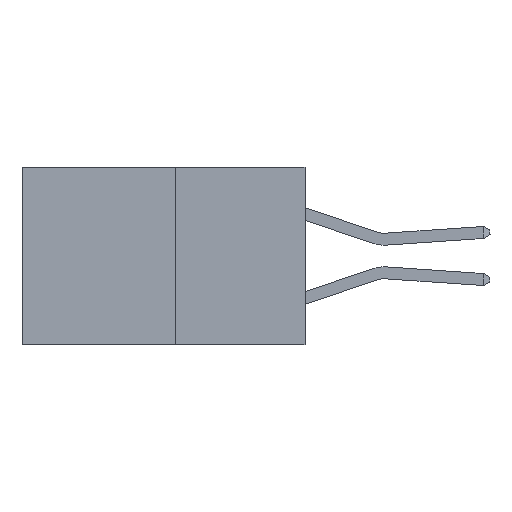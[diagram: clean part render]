
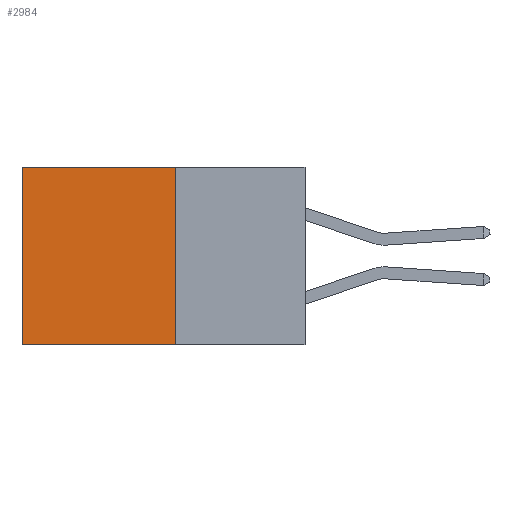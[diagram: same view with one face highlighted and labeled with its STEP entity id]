
A CAD part, left-side view. The second image highlights one B-rep face of the part: STEP entity #2984.
In plain terms, the highlighted planar face has unit normal (-1, 0, 0).
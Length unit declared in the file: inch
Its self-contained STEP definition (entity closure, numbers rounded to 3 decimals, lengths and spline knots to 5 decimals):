
#2 = AXIS2_PLACEMENT_3D ( 'NONE', #8184, #1617, #2459 ) ;
#181 = EDGE_CURVE ( 'NONE', #7901, #4941, #1417, .T. ) ;
#706 = CARTESIAN_POINT ( 'NONE',  ( 0.277, 0.27, 0. ) ) ;
#713 = DIRECTION ( 'NONE',  ( 0., 1., 0. ) ) ;
#1417 = LINE ( 'NONE', #7756, #6784 ) ;
#1617 = DIRECTION ( 'NONE',  ( 1., 0., 0. ) ) ;
#2149 = VECTOR ( 'NONE', #7917, 39.37008 ) ;
#2459 = DIRECTION ( 'NONE',  ( 0., 0., -1. ) ) ;
#2634 = DIRECTION ( 'NONE',  ( 0., 1., 0. ) ) ;
#2793 = VECTOR ( 'NONE', #4096, 39.37008 ) ;
#2984 = ADVANCED_FACE ( 'NONE', ( #8153 ), #8098, .F. ) ;
#3039 = LINE ( 'NONE', #4052, #2793 ) ;
#3084 = EDGE_LOOP ( 'NONE', ( #10181, #9084, #7384, #6349 ) ) ;
#4052 = CARTESIAN_POINT ( 'NONE',  ( 0.277, 0.27, -0.37 ) ) ;
#4096 = DIRECTION ( 'NONE',  ( 0., 0., -1. ) ) ;
#4941 = VERTEX_POINT ( 'NONE', #8812 ) ;
#5738 = CARTESIAN_POINT ( 'NONE',  ( 0.277, 0.59, 0. ) ) ;
#6165 = VERTEX_POINT ( 'NONE', #5738 ) ;
#6349 = ORIENTED_EDGE ( 'NONE', *, *, #7109, .T. ) ;
#6784 = VECTOR ( 'NONE', #2634, 39.37008 ) ;
#6865 = LINE ( 'NONE', #7895, #2149 ) ;
#7109 = EDGE_CURVE ( 'NONE', #9878, #6165, #9090, .T. ) ;
#7384 = ORIENTED_EDGE ( 'NONE', *, *, #8649, .F. ) ;
#7756 = CARTESIAN_POINT ( 'NONE',  ( 0.277, 0.27, -0.37 ) ) ;
#7895 = CARTESIAN_POINT ( 'NONE',  ( 0.277, 0.59, -0.37 ) ) ;
#7901 = VERTEX_POINT ( 'NONE', #9491 ) ;
#7917 = DIRECTION ( 'NONE',  ( 0., 0., -1. ) ) ;
#8081 = EDGE_CURVE ( 'NONE', #6165, #4941, #6865, .T. ) ;
#8098 = PLANE ( 'NONE',  #2 ) ;
#8153 = FACE_OUTER_BOUND ( 'NONE', #3084, .T. ) ;
#8184 = CARTESIAN_POINT ( 'NONE',  ( 0.277, 0.27, -0.37 ) ) ;
#8303 = CARTESIAN_POINT ( 'NONE',  ( 0.277, 0.27, 0. ) ) ;
#8649 = EDGE_CURVE ( 'NONE', #9878, #7901, #3039, .T. ) ;
#8812 = CARTESIAN_POINT ( 'NONE',  ( 0.277, 0.59, -0.37 ) ) ;
#8842 = VECTOR ( 'NONE', #713, 39.37008 ) ;
#9084 = ORIENTED_EDGE ( 'NONE', *, *, #181, .F. ) ;
#9090 = LINE ( 'NONE', #706, #8842 ) ;
#9491 = CARTESIAN_POINT ( 'NONE',  ( 0.277, 0.27, -0.37 ) ) ;
#9878 = VERTEX_POINT ( 'NONE', #8303 ) ;
#10181 = ORIENTED_EDGE ( 'NONE', *, *, #8081, .T. ) ;
